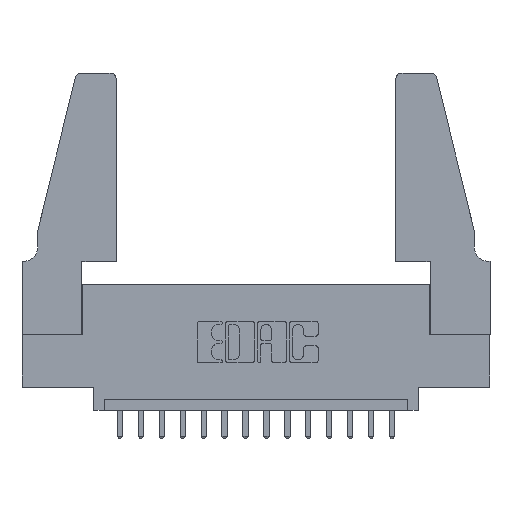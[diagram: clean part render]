
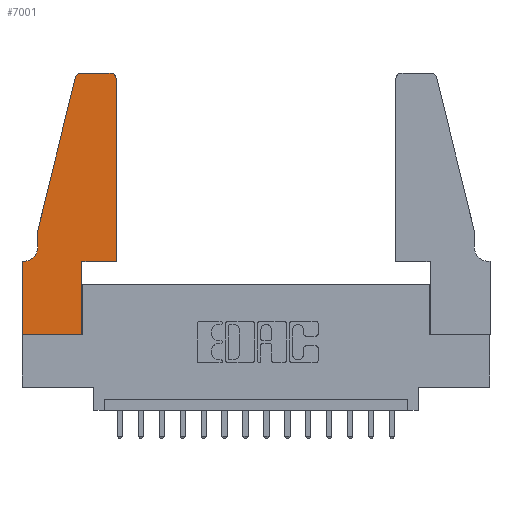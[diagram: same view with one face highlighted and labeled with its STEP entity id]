
A CAD part, top view. The second image highlights one B-rep face of the part: STEP entity #7001.
In plain terms, the highlighted planar face has unit normal (0, 0, 1).
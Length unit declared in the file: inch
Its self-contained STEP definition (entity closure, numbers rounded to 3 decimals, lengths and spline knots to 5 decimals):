
#59 = LINE ( 'NONE', #4075, #4285 ) ;
#540 = DIRECTION ( 'NONE',  ( 1., 0., 0. ) ) ;
#549 = CARTESIAN_POINT ( 'NONE',  ( 0.4505, 0.35, 0.37 ) ) ;
#922 = CARTESIAN_POINT ( 'NONE',  ( 0.284, 1.22, 0.37 ) ) ;
#1040 = FACE_OUTER_BOUND ( 'NONE', #7427, .T. ) ;
#1052 = DIRECTION ( 'NONE',  ( 0., 0., -1. ) ) ;
#1151 = VERTEX_POINT ( 'NONE', #11912 ) ;
#1662 = CARTESIAN_POINT ( 'NONE',  ( 0., 0.35, 0.37 ) ) ;
#1846 = EDGE_CURVE ( 'NONE', #11886, #2078, #3092, .T. ) ;
#1885 = CIRCLE ( 'NONE', #4810, 0.03 ) ;
#1970 = CARTESIAN_POINT ( 'NONE',  ( 0., 0.35, 0.37 ) ) ;
#2078 = VERTEX_POINT ( 'NONE', #10914 ) ;
#2458 = CARTESIAN_POINT ( 'NONE',  ( 0.0055, 0.35, 0.37 ) ) ;
#2477 = VECTOR ( 'NONE', #12742, 39.37008 ) ;
#3092 = CIRCLE ( 'NONE', #15708, 0.03 ) ;
#3147 = CIRCLE ( 'NONE', #4167, 0.07 ) ;
#3159 = CARTESIAN_POINT ( 'NONE',  ( 0.2865, 0., 0.37 ) ) ;
#3342 = EDGE_CURVE ( 'NONE', #10861, #11037, #8659, .T. ) ;
#3372 = DIRECTION ( 'NONE',  ( 1., 0., 0. ) ) ;
#3890 = CARTESIAN_POINT ( 'NONE',  ( 0., 0., 0.37 ) ) ;
#3891 = VERTEX_POINT ( 'NONE', #10252 ) ;
#4075 = CARTESIAN_POINT ( 'NONE',  ( 0.4505, 0.35, 0.37 ) ) ;
#4167 = AXIS2_PLACEMENT_3D ( 'NONE', #10089, #1052, #8615 ) ;
#4285 = VECTOR ( 'NONE', #13029, 39.37008 ) ;
#4349 = ORIENTED_EDGE ( 'NONE', *, *, #5875, .T. ) ;
#4398 = DIRECTION ( 'NONE',  ( -1., 0., 0. ) ) ;
#4434 = LINE ( 'NONE', #6218, #5210 ) ;
#4456 = EDGE_CURVE ( 'NONE', #1151, #10561, #10438, .T. ) ;
#4762 = LINE ( 'NONE', #10551, #7531 ) ;
#4810 = AXIS2_PLACEMENT_3D ( 'NONE', #922, #8432, #5952 ) ;
#4915 = ORIENTED_EDGE ( 'NONE', *, *, #11451, .T. ) ;
#4919 = DIRECTION ( 'NONE',  ( 0., 1., 0. ) ) ;
#5099 = ORIENTED_EDGE ( 'NONE', *, *, #8782, .T. ) ;
#5210 = VECTOR ( 'NONE', #10167, 39.37008 ) ;
#5374 = ORIENTED_EDGE ( 'NONE', *, *, #13610, .T. ) ;
#5377 = VECTOR ( 'NONE', #9147, 39.37008 ) ;
#5639 = EDGE_CURVE ( 'NONE', #6409, #1151, #1885, .T. ) ;
#5795 = VECTOR ( 'NONE', #9050, 39.37008 ) ;
#5875 = EDGE_CURVE ( 'NONE', #6341, #15565, #59, .T. ) ;
#5930 = EDGE_CURVE ( 'NONE', #15565, #11886, #8440, .T. ) ;
#5952 = DIRECTION ( 'NONE',  ( 1., 0., 0. ) ) ;
#6218 = CARTESIAN_POINT ( 'NONE',  ( 0., 0., 0.37 ) ) ;
#6341 = VERTEX_POINT ( 'NONE', #13807 ) ;
#6409 = VERTEX_POINT ( 'NONE', #10989 ) ;
#6433 = VECTOR ( 'NONE', #4919, 39.37008 ) ;
#6820 = EDGE_CURVE ( 'NONE', #11037, #3891, #4434, .T. ) ;
#6836 = CARTESIAN_POINT ( 'NONE',  ( 0.4205, 1.22, 0.37 ) ) ;
#6858 = CARTESIAN_POINT ( 'NONE',  ( 0.2865, 0.35, 0.37 ) ) ;
#6998 = ORIENTED_EDGE ( 'NONE', *, *, #5639, .T. ) ;
#7001 = ADVANCED_FACE ( 'NONE', ( #1040 ), #16259, .T. ) ;
#7411 = CARTESIAN_POINT ( 'NONE',  ( 0.0755, 0.42, 0.37 ) ) ;
#7427 = EDGE_LOOP ( 'NONE', ( #5374, #6998, #11885, #5099, #15600, #8123, #12967, #12729, #4915, #4349, #14671, #8511 ) ) ;
#7488 = VERTEX_POINT ( 'NONE', #7411 ) ;
#7531 = VECTOR ( 'NONE', #13053, 39.37008 ) ;
#7798 = DIRECTION ( 'NONE',  ( -1., 0., 0. ) ) ;
#8123 = ORIENTED_EDGE ( 'NONE', *, *, #3342, .T. ) ;
#8432 = DIRECTION ( 'NONE',  ( 0., 0., 1. ) ) ;
#8440 = LINE ( 'NONE', #14123, #6433 ) ;
#8511 = ORIENTED_EDGE ( 'NONE', *, *, #1846, .T. ) ;
#8615 = DIRECTION ( 'NONE',  ( -1., 0., 0. ) ) ;
#8658 = VERTEX_POINT ( 'NONE', #3159 ) ;
#8659 = LINE ( 'NONE', #10288, #11914 ) ;
#8782 = EDGE_CURVE ( 'NONE', #10561, #7488, #4762, .T. ) ;
#8828 = CARTESIAN_POINT ( 'NONE',  ( 0.0755, 0.5, 0.37 ) ) ;
#8965 = LINE ( 'NONE', #14696, #11777 ) ;
#9050 = DIRECTION ( 'NONE',  ( -0.239, -0.971, 0. ) ) ;
#9147 = DIRECTION ( 'NONE',  ( 0., 1., 0. ) ) ;
#9999 = LINE ( 'NONE', #6858, #5377 ) ;
#10089 = CARTESIAN_POINT ( 'NONE',  ( 0.0055, 0.42, 0.37 ) ) ;
#10167 = DIRECTION ( 'NONE',  ( 0., -1., 0. ) ) ;
#10252 = CARTESIAN_POINT ( 'NONE',  ( 0., 0., 0.37 ) ) ;
#10288 = CARTESIAN_POINT ( 'NONE',  ( 0.0755, 0.35, 0.37 ) ) ;
#10438 = LINE ( 'NONE', #10443, #5795 ) ;
#10440 = CARTESIAN_POINT ( 'NONE',  ( 0.4505, 1.22, 0.37 ) ) ;
#10443 = CARTESIAN_POINT ( 'NONE',  ( 0.0755, 0.5, 0.37 ) ) ;
#10551 = CARTESIAN_POINT ( 'NONE',  ( 0.0755, 0.5, 0.37 ) ) ;
#10561 = VERTEX_POINT ( 'NONE', #8828 ) ;
#10861 = VERTEX_POINT ( 'NONE', #2458 ) ;
#10914 = CARTESIAN_POINT ( 'NONE',  ( 0.4205, 1.25, 0.37 ) ) ;
#10989 = CARTESIAN_POINT ( 'NONE',  ( 0.284, 1.25, 0.37 ) ) ;
#11037 = VERTEX_POINT ( 'NONE', #1662 ) ;
#11451 = EDGE_CURVE ( 'NONE', #8658, #6341, #9999, .T. ) ;
#11777 = VECTOR ( 'NONE', #4398, 39.37008 ) ;
#11885 = ORIENTED_EDGE ( 'NONE', *, *, #4456, .T. ) ;
#11886 = VERTEX_POINT ( 'NONE', #10440 ) ;
#11912 = CARTESIAN_POINT ( 'NONE',  ( 0.25487, 1.22718, 0.37 ) ) ;
#11914 = VECTOR ( 'NONE', #7798, 39.37008 ) ;
#12729 = ORIENTED_EDGE ( 'NONE', *, *, #16288, .T. ) ;
#12742 = DIRECTION ( 'NONE',  ( 1., 0., 0. ) ) ;
#12967 = ORIENTED_EDGE ( 'NONE', *, *, #6820, .T. ) ;
#13029 = DIRECTION ( 'NONE',  ( 1., 0., 0. ) ) ;
#13053 = DIRECTION ( 'NONE',  ( 0., -1., 0. ) ) ;
#13610 = EDGE_CURVE ( 'NONE', #2078, #6409, #8965, .T. ) ;
#13807 = CARTESIAN_POINT ( 'NONE',  ( 0.2865, 0.35, 0.37 ) ) ;
#13951 = EDGE_CURVE ( 'NONE', #7488, #10861, #3147, .T. ) ;
#14123 = CARTESIAN_POINT ( 'NONE',  ( 0.4505, 0.35, 0.37 ) ) ;
#14529 = LINE ( 'NONE', #3890, #2477 ) ;
#14671 = ORIENTED_EDGE ( 'NONE', *, *, #5930, .T. ) ;
#14696 = CARTESIAN_POINT ( 'NONE',  ( 0.2605, 1.25, 0.37 ) ) ;
#14775 = DIRECTION ( 'NONE',  ( 0., 0., 1. ) ) ;
#14864 = DIRECTION ( 'NONE',  ( 0., 0., 1. ) ) ;
#15565 = VERTEX_POINT ( 'NONE', #549 ) ;
#15600 = ORIENTED_EDGE ( 'NONE', *, *, #13951, .T. ) ;
#15708 = AXIS2_PLACEMENT_3D ( 'NONE', #6836, #14775, #540 ) ;
#16124 = AXIS2_PLACEMENT_3D ( 'NONE', #1970, #14864, #3372 ) ;
#16259 = PLANE ( 'NONE',  #16124 ) ;
#16288 = EDGE_CURVE ( 'NONE', #3891, #8658, #14529, .T. ) ;
